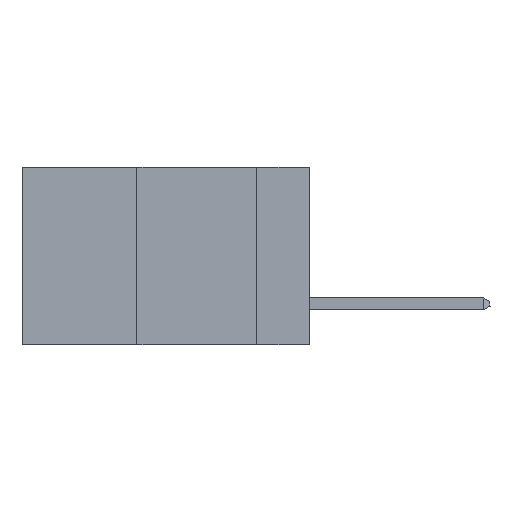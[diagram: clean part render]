
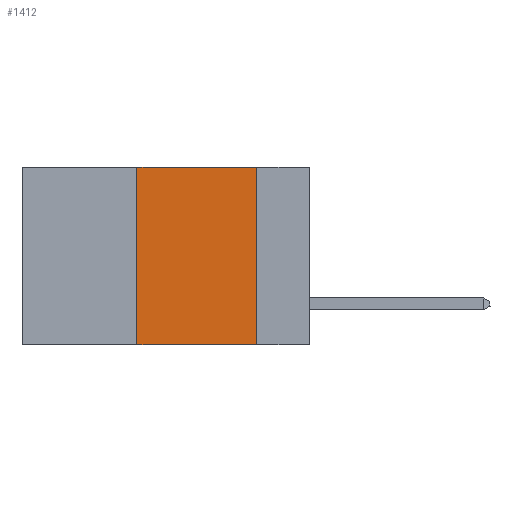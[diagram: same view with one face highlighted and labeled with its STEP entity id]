
A CAD part, left-side view. The second image highlights one B-rep face of the part: STEP entity #1412.
In plain terms, the highlighted planar face has unit normal (-1, 0, 0).
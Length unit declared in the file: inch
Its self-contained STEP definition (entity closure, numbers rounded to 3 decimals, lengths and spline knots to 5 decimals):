
#190 = CARTESIAN_POINT ( 'NONE',  ( 0., 0.11, 0. ) ) ;
#687 = VERTEX_POINT ( 'NONE', #4606 ) ;
#772 = ORIENTED_EDGE ( 'NONE', *, *, #1024, .F. ) ;
#1024 = EDGE_CURVE ( 'NONE', #28815, #3688, #10006, .T. ) ;
#1147 = LINE ( 'NONE', #39075, #1609 ) ;
#1412 = ADVANCED_FACE ( 'NONE', ( #15308 ), #8902, .F. ) ;
#1609 = VECTOR ( 'NONE', #26593, 39.37008 ) ;
#2126 = LINE ( 'NONE', #7614, #34346 ) ;
#2908 = DIRECTION ( 'NONE',  ( 0., 0., -1. ) ) ;
#3033 = DIRECTION ( 'NONE',  ( 1., 0., 0. ) ) ;
#3484 = DIRECTION ( 'NONE',  ( 0., 0., -1. ) ) ;
#3688 = VERTEX_POINT ( 'NONE', #39117 ) ;
#4606 = CARTESIAN_POINT ( 'NONE',  ( 0., 0.36, 0. ) ) ;
#6599 = VERTEX_POINT ( 'NONE', #11927 ) ;
#7614 = CARTESIAN_POINT ( 'NONE',  ( 0., 0.6, -0.37 ) ) ;
#8679 = DIRECTION ( 'NONE',  ( 0., -1., 0. ) ) ;
#8902 = PLANE ( 'NONE',  #18057 ) ;
#9494 = CARTESIAN_POINT ( 'NONE',  ( 0., 0.11, 0. ) ) ;
#10006 = LINE ( 'NONE', #9494, #38309 ) ;
#10083 = EDGE_CURVE ( 'NONE', #6599, #687, #1147, .T. ) ;
#10904 = ORIENTED_EDGE ( 'NONE', *, *, #26357, .F. ) ;
#11927 = CARTESIAN_POINT ( 'NONE',  ( 0., 0.36, -0.37 ) ) ;
#14665 = CARTESIAN_POINT ( 'NONE',  ( 0., 0.6, 0. ) ) ;
#15308 = FACE_OUTER_BOUND ( 'NONE', #19484, .T. ) ;
#18057 = AXIS2_PLACEMENT_3D ( 'NONE', #40295, #3033, #2908 ) ;
#19484 = EDGE_LOOP ( 'NONE', ( #772, #10904, #31113, #21134 ) ) ;
#21134 = ORIENTED_EDGE ( 'NONE', *, *, #21671, .T. ) ;
#21671 = EDGE_CURVE ( 'NONE', #6599, #3688, #2126, .T. ) ;
#26357 = EDGE_CURVE ( 'NONE', #687, #28815, #36081, .T. ) ;
#26593 = DIRECTION ( 'NONE',  ( 0., 0., 1. ) ) ;
#28815 = VERTEX_POINT ( 'NONE', #190 ) ;
#31113 = ORIENTED_EDGE ( 'NONE', *, *, #10083, .F. ) ;
#34148 = VECTOR ( 'NONE', #8679, 39.37008 ) ;
#34346 = VECTOR ( 'NONE', #39004, 39.37008 ) ;
#36081 = LINE ( 'NONE', #14665, #34148 ) ;
#38309 = VECTOR ( 'NONE', #3484, 39.37008 ) ;
#39004 = DIRECTION ( 'NONE',  ( 0., -1., 0. ) ) ;
#39075 = CARTESIAN_POINT ( 'NONE',  ( 0., 0.36, 0. ) ) ;
#39117 = CARTESIAN_POINT ( 'NONE',  ( 0., 0.11, -0.37 ) ) ;
#40295 = CARTESIAN_POINT ( 'NONE',  ( 0., 0.6, 0. ) ) ;
